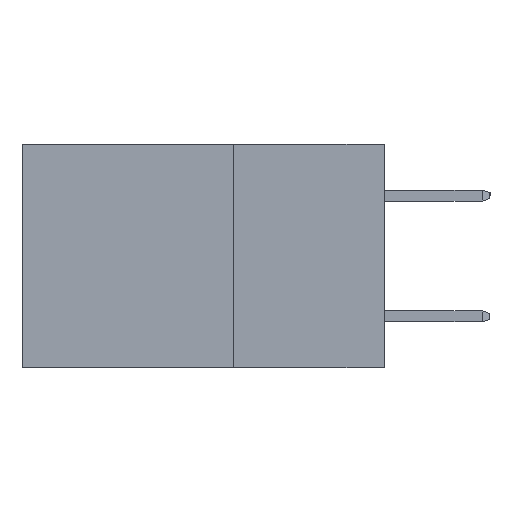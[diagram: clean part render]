
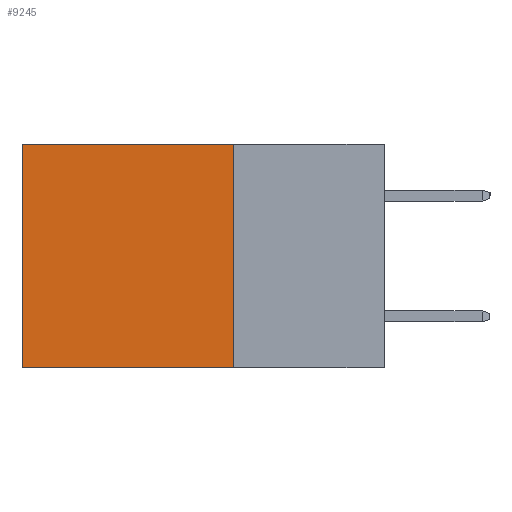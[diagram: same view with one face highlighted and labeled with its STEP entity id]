
A CAD part, left-side view. The second image highlights one B-rep face of the part: STEP entity #9245.
In plain terms, the highlighted planar face has unit normal (-1, 0, 0).
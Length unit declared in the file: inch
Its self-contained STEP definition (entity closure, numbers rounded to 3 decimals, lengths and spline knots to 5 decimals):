
#42 = DIRECTION ( 'NONE',  ( 0., 0., -1. ) ) ;
#445 = VERTEX_POINT ( 'NONE', #862 ) ;
#531 = CARTESIAN_POINT ( 'NONE',  ( 0.2615, 0.6, -0.37 ) ) ;
#568 = EDGE_CURVE ( 'NONE', #445, #11750, #6358, .T. ) ;
#862 = CARTESIAN_POINT ( 'NONE',  ( 0.2615, 0.6, 0. ) ) ;
#1231 = ORIENTED_EDGE ( 'NONE', *, *, #5236, .F. ) ;
#1427 = FACE_OUTER_BOUND ( 'NONE', #6560, .T. ) ;
#1723 = VECTOR ( 'NONE', #42, 39.37008 ) ;
#2245 = CARTESIAN_POINT ( 'NONE',  ( 0.2615, 0.25, -0.37 ) ) ;
#2723 = DIRECTION ( 'NONE',  ( 0., 1., 0. ) ) ;
#2830 = PLANE ( 'NONE',  #7588 ) ;
#2932 = VECTOR ( 'NONE', #10514, 39.37008 ) ;
#3270 = LINE ( 'NONE', #2245, #2932 ) ;
#3564 = EDGE_CURVE ( 'NONE', #5109, #445, #4635, .T. ) ;
#4635 = LINE ( 'NONE', #4700, #6383 ) ;
#4700 = CARTESIAN_POINT ( 'NONE',  ( 0.2615, 0.25, 0. ) ) ;
#4977 = VECTOR ( 'NONE', #9897, 39.37008 ) ;
#5109 = VERTEX_POINT ( 'NONE', #5234 ) ;
#5234 = CARTESIAN_POINT ( 'NONE',  ( 0.2615, 0.25, 0. ) ) ;
#5236 = EDGE_CURVE ( 'NONE', #5109, #6709, #3270, .T. ) ;
#5962 = CARTESIAN_POINT ( 'NONE',  ( 0.2615, 0.25, -0.37 ) ) ;
#6358 = LINE ( 'NONE', #11364, #1723 ) ;
#6383 = VECTOR ( 'NONE', #2723, 39.37008 ) ;
#6560 = EDGE_LOOP ( 'NONE', ( #10958, #11995, #1231, #7784 ) ) ;
#6709 = VERTEX_POINT ( 'NONE', #8195 ) ;
#7449 = EDGE_CURVE ( 'NONE', #6709, #11750, #10106, .T. ) ;
#7588 = AXIS2_PLACEMENT_3D ( 'NONE', #5962, #11038, #11795 ) ;
#7784 = ORIENTED_EDGE ( 'NONE', *, *, #3564, .T. ) ;
#8195 = CARTESIAN_POINT ( 'NONE',  ( 0.2615, 0.25, -0.37 ) ) ;
#8820 = CARTESIAN_POINT ( 'NONE',  ( 0.2615, 0.25, -0.37 ) ) ;
#9245 = ADVANCED_FACE ( 'NONE', ( #1427 ), #2830, .F. ) ;
#9897 = DIRECTION ( 'NONE',  ( 0., 1., 0. ) ) ;
#10106 = LINE ( 'NONE', #8820, #4977 ) ;
#10514 = DIRECTION ( 'NONE',  ( 0., 0., -1. ) ) ;
#10958 = ORIENTED_EDGE ( 'NONE', *, *, #568, .T. ) ;
#11038 = DIRECTION ( 'NONE',  ( 1., 0., 0. ) ) ;
#11364 = CARTESIAN_POINT ( 'NONE',  ( 0.2615, 0.6, -0.37 ) ) ;
#11750 = VERTEX_POINT ( 'NONE', #531 ) ;
#11795 = DIRECTION ( 'NONE',  ( 0., 0., -1. ) ) ;
#11995 = ORIENTED_EDGE ( 'NONE', *, *, #7449, .F. ) ;
